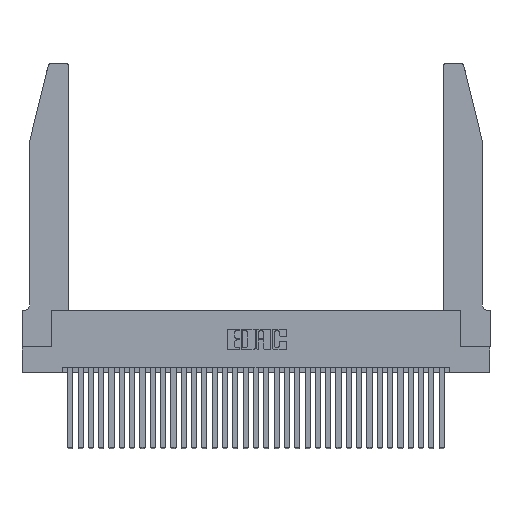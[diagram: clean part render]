
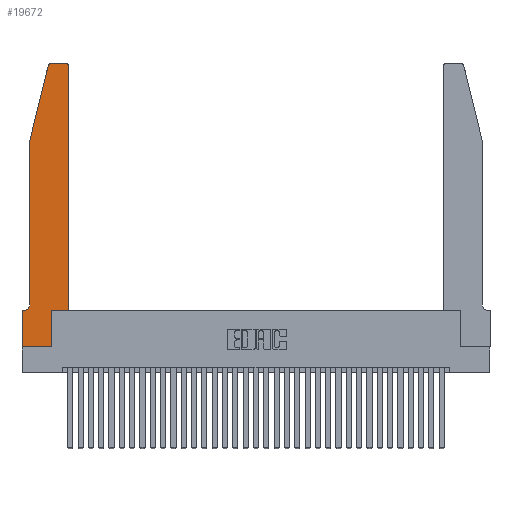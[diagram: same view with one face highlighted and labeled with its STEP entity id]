
A CAD part, top view. The second image highlights one B-rep face of the part: STEP entity #19672.
In plain terms, the highlighted planar face has unit normal (0, 0, 1).
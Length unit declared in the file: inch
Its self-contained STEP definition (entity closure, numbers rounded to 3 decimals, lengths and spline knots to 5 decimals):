
#182 = VECTOR ( 'NONE', #12700, 39.37008 ) ;
#698 = VERTEX_POINT ( 'NONE', #15779 ) ;
#891 = AXIS2_PLACEMENT_3D ( 'NONE', #14219, #6462, #17283 ) ;
#1390 = CARTESIAN_POINT ( 'NONE',  ( 0.0755, 2., 0.37 ) ) ;
#1749 = EDGE_CURVE ( 'NONE', #698, #31512, #18451, .T. ) ;
#2129 = FACE_OUTER_BOUND ( 'NONE', #9425, .T. ) ;
#2463 = ORIENTED_EDGE ( 'NONE', *, *, #27237, .T. ) ;
#2660 = DIRECTION ( 'NONE',  ( 0., -1., 0. ) ) ;
#2693 = EDGE_CURVE ( 'NONE', #2778, #2789, #6288, .T. ) ;
#2778 = VERTEX_POINT ( 'NONE', #3210 ) ;
#2789 = VERTEX_POINT ( 'NONE', #6010 ) ;
#3210 = CARTESIAN_POINT ( 'NONE',  ( 0.4505, 0.35, 0.37 ) ) ;
#3904 = CARTESIAN_POINT ( 'NONE',  ( 0., 0.35, 0.37 ) ) ;
#4059 = ORIENTED_EDGE ( 'NONE', *, *, #1749, .T. ) ;
#4450 = VERTEX_POINT ( 'NONE', #7061 ) ;
#4510 = CARTESIAN_POINT ( 'NONE',  ( 0.284, 2.75, 0.37 ) ) ;
#5750 = EDGE_CURVE ( 'NONE', #28403, #17266, #29831, .T. ) ;
#6010 = CARTESIAN_POINT ( 'NONE',  ( 0.4505, 2.72, 0.37 ) ) ;
#6288 = LINE ( 'NONE', #12737, #21252 ) ;
#6462 = DIRECTION ( 'NONE',  ( 0., 0., -1. ) ) ;
#6478 = EDGE_CURVE ( 'NONE', #21797, #25704, #19844, .T. ) ;
#6531 = ORIENTED_EDGE ( 'NONE', *, *, #9744, .T. ) ;
#6725 = AXIS2_PLACEMENT_3D ( 'NONE', #16171, #7911, #29289 ) ;
#7061 = CARTESIAN_POINT ( 'NONE',  ( 0., 0., 0.37 ) ) ;
#7198 = EDGE_CURVE ( 'NONE', #17266, #4450, #14853, .T. ) ;
#7854 = VERTEX_POINT ( 'NONE', #22482 ) ;
#7911 = DIRECTION ( 'NONE',  ( 0., 0., 1. ) ) ;
#9156 = DIRECTION ( 'NONE',  ( 1., 0., 0. ) ) ;
#9425 = EDGE_LOOP ( 'NONE', ( #33599, #15037, #4059, #21228, #15256, #17258, #30275, #29911, #28862, #6531, #14011, #2463 ) ) ;
#9532 = CARTESIAN_POINT ( 'NONE',  ( 0.4505, 0.35, 0.37 ) ) ;
#9744 = EDGE_CURVE ( 'NONE', #32783, #2778, #21907, .T. ) ;
#10169 = AXIS2_PLACEMENT_3D ( 'NONE', #21884, #18884, #13539 ) ;
#10594 = CIRCLE ( 'NONE', #891, 0.07 ) ;
#12310 = VERTEX_POINT ( 'NONE', #15399 ) ;
#12693 = LINE ( 'NONE', #1390, #33030 ) ;
#12700 = DIRECTION ( 'NONE',  ( -0.239, -0.971, 0. ) ) ;
#12737 = CARTESIAN_POINT ( 'NONE',  ( 0.4505, 0.35, 0.37 ) ) ;
#13340 = AXIS2_PLACEMENT_3D ( 'NONE', #3904, #16911, #22486 ) ;
#13539 = DIRECTION ( 'NONE',  ( 1., 0., 0. ) ) ;
#14011 = ORIENTED_EDGE ( 'NONE', *, *, #2693, .T. ) ;
#14219 = CARTESIAN_POINT ( 'NONE',  ( 0.0055, 0.42, 0.37 ) ) ;
#14392 = VECTOR ( 'NONE', #2660, 39.37008 ) ;
#14853 = LINE ( 'NONE', #28768, #14392 ) ;
#14904 = VECTOR ( 'NONE', #9156, 39.37008 ) ;
#14994 = DIRECTION ( 'NONE',  ( -1., 0., 0. ) ) ;
#15037 = ORIENTED_EDGE ( 'NONE', *, *, #32598, .T. ) ;
#15256 = ORIENTED_EDGE ( 'NONE', *, *, #31665, .T. ) ;
#15291 = DIRECTION ( 'NONE',  ( -1., 0., 0. ) ) ;
#15399 = CARTESIAN_POINT ( 'NONE',  ( 0.0755, 0.42, 0.37 ) ) ;
#15743 = VECTOR ( 'NONE', #15291, 39.37008 ) ;
#15779 = CARTESIAN_POINT ( 'NONE',  ( 0.25487, 2.72718, 0.37 ) ) ;
#15931 = CIRCLE ( 'NONE', #6725, 0.03 ) ;
#16171 = CARTESIAN_POINT ( 'NONE',  ( 0.284, 2.72, 0.37 ) ) ;
#16911 = DIRECTION ( 'NONE',  ( 0., 0., 1. ) ) ;
#17258 = ORIENTED_EDGE ( 'NONE', *, *, #5750, .T. ) ;
#17266 = VERTEX_POINT ( 'NONE', #29127 ) ;
#17283 = DIRECTION ( 'NONE',  ( -1., 0., 0. ) ) ;
#17879 = DIRECTION ( 'NONE',  ( 0., 1., 0. ) ) ;
#18451 = LINE ( 'NONE', #20379, #182 ) ;
#18884 = DIRECTION ( 'NONE',  ( 0., 0., 1. ) ) ;
#19665 = LINE ( 'NONE', #28707, #29637 ) ;
#19672 = ADVANCED_FACE ( 'NONE', ( #2129 ), #27579, .T. ) ;
#19844 = LINE ( 'NONE', #20188, #29805 ) ;
#20188 = CARTESIAN_POINT ( 'NONE',  ( 0.2605, 2.75, 0.37 ) ) ;
#20379 = CARTESIAN_POINT ( 'NONE',  ( 0.0755, 2., 0.37 ) ) ;
#21228 = ORIENTED_EDGE ( 'NONE', *, *, #31130, .T. ) ;
#21252 = VECTOR ( 'NONE', #17879, 39.37008 ) ;
#21797 = VERTEX_POINT ( 'NONE', #23983 ) ;
#21884 = CARTESIAN_POINT ( 'NONE',  ( 0.4205, 2.72, 0.37 ) ) ;
#21907 = LINE ( 'NONE', #9532, #14904 ) ;
#21939 = CARTESIAN_POINT ( 'NONE',  ( 0.2865, 0.35, 0.37 ) ) ;
#22482 = CARTESIAN_POINT ( 'NONE',  ( 0.2865, 0., 0.37 ) ) ;
#22486 = DIRECTION ( 'NONE',  ( 1., 0., 0. ) ) ;
#23096 = LINE ( 'NONE', #31875, #28067 ) ;
#23983 = CARTESIAN_POINT ( 'NONE',  ( 0.4205, 2.75, 0.37 ) ) ;
#25704 = VERTEX_POINT ( 'NONE', #4510 ) ;
#26339 = EDGE_CURVE ( 'NONE', #4450, #7854, #19665, .T. ) ;
#27237 = EDGE_CURVE ( 'NONE', #2789, #21797, #27502, .T. ) ;
#27502 = CIRCLE ( 'NONE', #10169, 0.03 ) ;
#27579 = PLANE ( 'NONE',  #13340 ) ;
#28067 = VECTOR ( 'NONE', #31778, 39.37008 ) ;
#28403 = VERTEX_POINT ( 'NONE', #34127 ) ;
#28707 = CARTESIAN_POINT ( 'NONE',  ( 0., 0., 0.37 ) ) ;
#28768 = CARTESIAN_POINT ( 'NONE',  ( 0., 0., 0.37 ) ) ;
#28862 = ORIENTED_EDGE ( 'NONE', *, *, #31434, .T. ) ;
#29127 = CARTESIAN_POINT ( 'NONE',  ( 0., 0.35, 0.37 ) ) ;
#29289 = DIRECTION ( 'NONE',  ( 1., 0., 0. ) ) ;
#29637 = VECTOR ( 'NONE', #30940, 39.37008 ) ;
#29805 = VECTOR ( 'NONE', #14994, 39.37008 ) ;
#29831 = LINE ( 'NONE', #32006, #15743 ) ;
#29911 = ORIENTED_EDGE ( 'NONE', *, *, #26339, .T. ) ;
#30275 = ORIENTED_EDGE ( 'NONE', *, *, #7198, .T. ) ;
#30940 = DIRECTION ( 'NONE',  ( 1., 0., 0. ) ) ;
#31130 = EDGE_CURVE ( 'NONE', #31512, #12310, #12693, .T. ) ;
#31434 = EDGE_CURVE ( 'NONE', #7854, #32783, #23096, .T. ) ;
#31512 = VERTEX_POINT ( 'NONE', #32663 ) ;
#31665 = EDGE_CURVE ( 'NONE', #12310, #28403, #10594, .T. ) ;
#31778 = DIRECTION ( 'NONE',  ( 0., 1., 0. ) ) ;
#31875 = CARTESIAN_POINT ( 'NONE',  ( 0.2865, 0.35, 0.37 ) ) ;
#32006 = CARTESIAN_POINT ( 'NONE',  ( 0.0755, 0.35, 0.37 ) ) ;
#32598 = EDGE_CURVE ( 'NONE', #25704, #698, #15931, .T. ) ;
#32663 = CARTESIAN_POINT ( 'NONE',  ( 0.0755, 2., 0.37 ) ) ;
#32783 = VERTEX_POINT ( 'NONE', #21939 ) ;
#32803 = DIRECTION ( 'NONE',  ( 0., -1., 0. ) ) ;
#33030 = VECTOR ( 'NONE', #32803, 39.37008 ) ;
#33599 = ORIENTED_EDGE ( 'NONE', *, *, #6478, .T. ) ;
#34127 = CARTESIAN_POINT ( 'NONE',  ( 0.0055, 0.35, 0.37 ) ) ;
